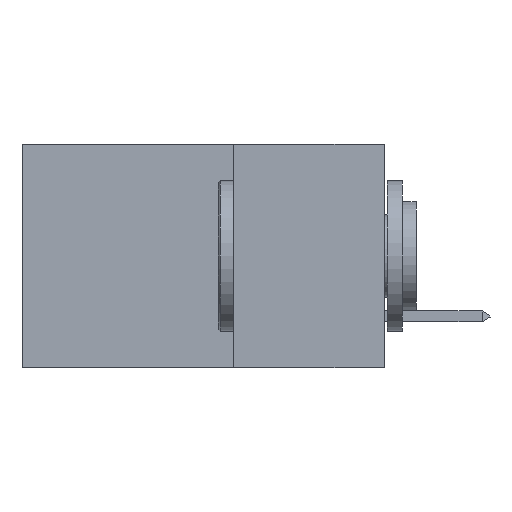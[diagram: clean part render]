
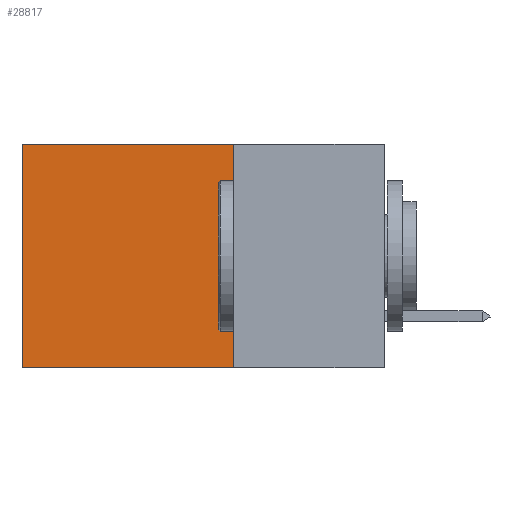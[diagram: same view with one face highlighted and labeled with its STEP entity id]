
A CAD part, left-side view. The second image highlights one B-rep face of the part: STEP entity #28817.
In plain terms, the highlighted planar face has unit normal (-1, 0, 0).
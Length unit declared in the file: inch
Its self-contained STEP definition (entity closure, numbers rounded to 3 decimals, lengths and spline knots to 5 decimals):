
#859 = LINE ( 'NONE', #8146, #34113 ) ;
#1010 = ORIENTED_EDGE ( 'NONE', *, *, #30976, .T. ) ;
#1455 = DIRECTION ( 'NONE',  ( 0., 0., -1. ) ) ;
#2092 = AXIS2_PLACEMENT_3D ( 'NONE', #18310, #30079, #1455 ) ;
#2723 = VERTEX_POINT ( 'NONE', #23318 ) ;
#3764 = EDGE_CURVE ( 'NONE', #16293, #15196, #20029, .T. ) ;
#4132 = DIRECTION ( 'NONE',  ( 0., 0., -1. ) ) ;
#7099 = EDGE_CURVE ( 'NONE', #2723, #36247, #31343, .T. ) ;
#7109 = DIRECTION ( 'NONE',  ( 0., 0., -1. ) ) ;
#8146 = CARTESIAN_POINT ( 'NONE',  ( 0.2875, 0.6, 0. ) ) ;
#10885 = CARTESIAN_POINT ( 'NONE',  ( 0.2875, 0.6, 0. ) ) ;
#13986 = EDGE_CURVE ( 'NONE', #2723, #16293, #34252, .T. ) ;
#14523 = VECTOR ( 'NONE', #26943, 39.37008 ) ;
#15196 = VERTEX_POINT ( 'NONE', #27296 ) ;
#15512 = EDGE_LOOP ( 'NONE', ( #1010, #35261, #30527, #18317 ) ) ;
#16293 = VERTEX_POINT ( 'NONE', #31803 ) ;
#17674 = CARTESIAN_POINT ( 'NONE',  ( 0.2875, 0.25, -0.37 ) ) ;
#18310 = CARTESIAN_POINT ( 'NONE',  ( 0.2875, 0.25, 0. ) ) ;
#18317 = ORIENTED_EDGE ( 'NONE', *, *, #7099, .T. ) ;
#20029 = LINE ( 'NONE', #17674, #21368 ) ;
#20174 = CARTESIAN_POINT ( 'NONE',  ( 0.2875, 0.25, 0. ) ) ;
#21368 = VECTOR ( 'NONE', #23601, 39.37008 ) ;
#22753 = FACE_OUTER_BOUND ( 'NONE', #15512, .T. ) ;
#23172 = VECTOR ( 'NONE', #4132, 39.37008 ) ;
#23318 = CARTESIAN_POINT ( 'NONE',  ( 0.2875, 0.25, 0. ) ) ;
#23601 = DIRECTION ( 'NONE',  ( 0., 1., 0. ) ) ;
#24212 = CARTESIAN_POINT ( 'NONE',  ( 0.2875, 0.25, 0. ) ) ;
#24247 = PLANE ( 'NONE',  #2092 ) ;
#26943 = DIRECTION ( 'NONE',  ( 0., 1., 0. ) ) ;
#27296 = CARTESIAN_POINT ( 'NONE',  ( 0.2875, 0.6, -0.37 ) ) ;
#28817 = ADVANCED_FACE ( 'NONE', ( #22753 ), #24247, .F. ) ;
#30079 = DIRECTION ( 'NONE',  ( 1., 0., 0. ) ) ;
#30527 = ORIENTED_EDGE ( 'NONE', *, *, #13986, .F. ) ;
#30976 = EDGE_CURVE ( 'NONE', #36247, #15196, #859, .T. ) ;
#31343 = LINE ( 'NONE', #24212, #14523 ) ;
#31803 = CARTESIAN_POINT ( 'NONE',  ( 0.2875, 0.25, -0.37 ) ) ;
#34113 = VECTOR ( 'NONE', #7109, 39.37008 ) ;
#34252 = LINE ( 'NONE', #20174, #23172 ) ;
#35261 = ORIENTED_EDGE ( 'NONE', *, *, #3764, .F. ) ;
#36247 = VERTEX_POINT ( 'NONE', #10885 ) ;
